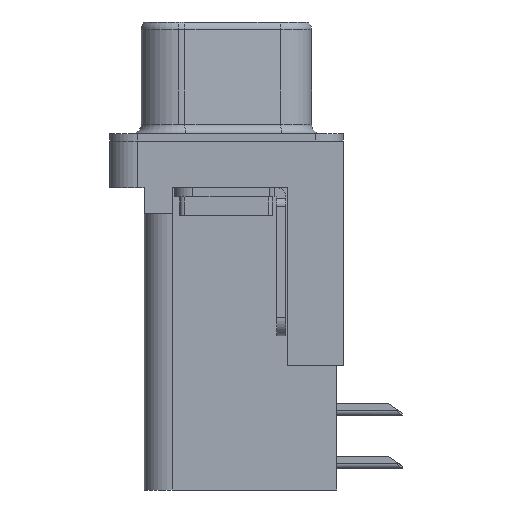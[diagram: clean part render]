
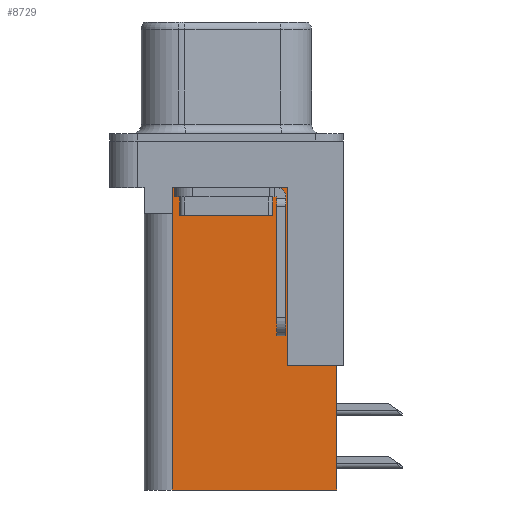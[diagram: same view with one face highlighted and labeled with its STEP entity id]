
A CAD part, left-side view. The second image highlights one B-rep face of the part: STEP entity #8729.
In plain terms, the highlighted planar face has unit normal (-1, 0, 0).
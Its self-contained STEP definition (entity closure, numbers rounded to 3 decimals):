
#166 = VECTOR ( 'NONE', #6045, 1000. ) ;
#988 = VECTOR ( 'NONE', #2101, 1000. ) ;
#1036 = LINE ( 'NONE', #6086, #3636 ) ;
#1727 = LINE ( 'NONE', #8256, #10849 ) ;
#1754 = CARTESIAN_POINT ( 'NONE',  ( 3.79, 0., -3.9 ) ) ;
#2002 = LINE ( 'NONE', #15973, #10709 ) ;
#2004 = ORIENTED_EDGE ( 'NONE', *, *, #14362, .F. ) ;
#2101 = DIRECTION ( 'NONE',  ( 0., 0., -1. ) ) ;
#2378 = ORIENTED_EDGE ( 'NONE', *, *, #7383, .F. ) ;
#2568 = LINE ( 'NONE', #1754, #5524 ) ;
#2825 = VERTEX_POINT ( 'NONE', #5193 ) ;
#2919 = DIRECTION ( 'NONE',  ( 0., 1., 0. ) ) ;
#3636 = VECTOR ( 'NONE', #7375, 1000. ) ;
#3779 = CARTESIAN_POINT ( 'NONE',  ( 3.79, 2.925, -3.9 ) ) ;
#4289 = DIRECTION ( 'NONE',  ( 0., 0., -1. ) ) ;
#4687 = VERTEX_POINT ( 'NONE', #3779 ) ;
#4756 = CARTESIAN_POINT ( 'NONE',  ( 3.79, -3.295, -18.76 ) ) ;
#4946 = CARTESIAN_POINT ( 'NONE',  ( 3.79, -3.295, -12.05 ) ) ;
#5193 = CARTESIAN_POINT ( 'NONE',  ( 3.79, 2.895, -2.5 ) ) ;
#5231 = ORIENTED_EDGE ( 'NONE', *, *, #10851, .T. ) ;
#5506 = VECTOR ( 'NONE', #4289, 1000. ) ;
#5509 = ORIENTED_EDGE ( 'NONE', *, *, #8781, .F. ) ;
#5522 = CARTESIAN_POINT ( 'NONE',  ( 3.79, -3.295, -2.5 ) ) ;
#5524 = VECTOR ( 'NONE', #12985, 1000. ) ;
#5681 = DIRECTION ( 'NONE',  ( 0., 0., 1. ) ) ;
#5950 = AXIS2_PLACEMENT_3D ( 'NONE', #9133, #10312, #2919 ) ;
#6008 = LINE ( 'NONE', #7270, #12117 ) ;
#6045 = DIRECTION ( 'NONE',  ( 0., 1., 0. ) ) ;
#6086 = CARTESIAN_POINT ( 'NONE',  ( 3.79, -6.295, -12.05 ) ) ;
#6149 = VERTEX_POINT ( 'NONE', #8259 ) ;
#6353 = EDGE_CURVE ( 'NONE', #12299, #2825, #2002, .T. ) ;
#7193 = CARTESIAN_POINT ( 'NONE',  ( 3.79, 2.895, -3.9 ) ) ;
#7210 = ORIENTED_EDGE ( 'NONE', *, *, #11157, .T. ) ;
#7270 = CARTESIAN_POINT ( 'NONE',  ( 3.79, -3.295, -18.76 ) ) ;
#7323 = EDGE_CURVE ( 'NONE', #2825, #11801, #14218, .T. ) ;
#7375 = DIRECTION ( 'NONE',  ( 0., 1., 0. ) ) ;
#7383 = EDGE_CURVE ( 'NONE', #6149, #7940, #10139, .T. ) ;
#7940 = VERTEX_POINT ( 'NONE', #15629 ) ;
#7943 = PLANE ( 'NONE',  #5950 ) ;
#8209 = EDGE_CURVE ( 'NONE', #11801, #4687, #2568, .T. ) ;
#8256 = CARTESIAN_POINT ( 'NONE',  ( 3.79, 2.925, -18.76 ) ) ;
#8259 = CARTESIAN_POINT ( 'NONE',  ( 3.79, -5.925, -18.76 ) ) ;
#8468 = DIRECTION ( 'NONE',  ( 0., 0., 1. ) ) ;
#8729 = ADVANCED_FACE ( 'NONE', ( #12046 ), #7943, .F. ) ;
#8781 = EDGE_CURVE ( 'NONE', #10509, #6149, #14554, .T. ) ;
#9133 = CARTESIAN_POINT ( 'NONE',  ( 3.79, -3.295, -18.76 ) ) ;
#9891 = DIRECTION ( 'NONE',  ( 0., 1., 0. ) ) ;
#10139 = LINE ( 'NONE', #4756, #166 ) ;
#10312 = DIRECTION ( 'NONE',  ( 1., 0., 0. ) ) ;
#10426 = EDGE_LOOP ( 'NONE', ( #11560, #15221, #13479, #2004, #2378, #5509, #5231, #7210 ) ) ;
#10509 = VERTEX_POINT ( 'NONE', #13855 ) ;
#10709 = VECTOR ( 'NONE', #9891, 1000. ) ;
#10849 = VECTOR ( 'NONE', #5681, 1000. ) ;
#10851 = EDGE_CURVE ( 'NONE', #10509, #11990, #1036, .T. ) ;
#11157 = EDGE_CURVE ( 'NONE', #11990, #12299, #6008, .T. ) ;
#11560 = ORIENTED_EDGE ( 'NONE', *, *, #6353, .T. ) ;
#11801 = VERTEX_POINT ( 'NONE', #7193 ) ;
#11990 = VERTEX_POINT ( 'NONE', #4946 ) ;
#12046 = FACE_OUTER_BOUND ( 'NONE', #10426, .T. ) ;
#12117 = VECTOR ( 'NONE', #8468, 1000. ) ;
#12299 = VERTEX_POINT ( 'NONE', #5522 ) ;
#12923 = CARTESIAN_POINT ( 'NONE',  ( 3.79, -5.925, -2. ) ) ;
#12985 = DIRECTION ( 'NONE',  ( 0., 1., 0. ) ) ;
#13479 = ORIENTED_EDGE ( 'NONE', *, *, #8209, .T. ) ;
#13855 = CARTESIAN_POINT ( 'NONE',  ( 3.79, -5.925, -12.05 ) ) ;
#14218 = LINE ( 'NONE', #15600, #988 ) ;
#14362 = EDGE_CURVE ( 'NONE', #7940, #4687, #1727, .T. ) ;
#14554 = LINE ( 'NONE', #12923, #5506 ) ;
#15221 = ORIENTED_EDGE ( 'NONE', *, *, #7323, .T. ) ;
#15600 = CARTESIAN_POINT ( 'NONE',  ( 3.79, 2.895, -3.9 ) ) ;
#15629 = CARTESIAN_POINT ( 'NONE',  ( 3.79, 2.925, -18.76 ) ) ;
#15973 = CARTESIAN_POINT ( 'NONE',  ( 3.79, -3.295, -2.5 ) ) ;
